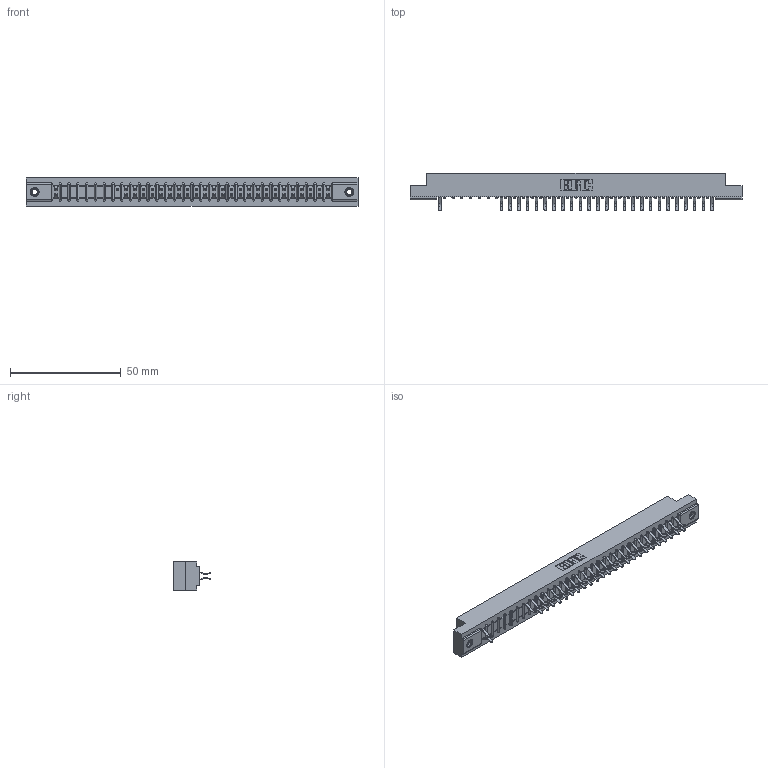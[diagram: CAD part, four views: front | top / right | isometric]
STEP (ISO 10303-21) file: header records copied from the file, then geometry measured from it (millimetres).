
FILE_DESCRIPTION (( 'STEP AP203' ), '1' );
FILE_NAME ('307-064-556-207.STEP', '2018-08-06T10:25:13', ( '' ), ( '' ), 'SwSTEP 2.0', 'SolidWorks 2016', '' );
FILE_SCHEMA (( 'CONFIG_CONTROL_DESIGN' ));
Length unit declared in the file: inch
Products named in the file (4): 307 Part_.156 Dia Mounting Holes; 307-290-001_556; 345-250-001_345-250-005-103; 307-064-556-207
Assembly tree (54 placements, depth 2):
  307-064-556-207
    307 Part_.156 Dia Mounting Holes
    307-290-001_556  x51
    345-250-001_345-250-005-103  x2
Bounding box: 149.81 x 16.97 x 12.7 mm (x, y, z)
Volume: 15668.5 mm3; surface area: 17763.1 mm2
Topology: 54 solids, 54 shells, 2891 faces, 8117 edges, 5246 vertices
Faces by surface type: plane 1863, cylinder 946, sphere 66, cone 12, torus 4
Entity records: 30563 total; most frequent: CARTESIAN_POINT 5042, ORIENTED_EDGE 5002, DIRECTION 4939, EDGE_CURVE 2501, LINE 1913, VECTOR 1913, VERTEX_POINT 1616, AXIS2_PLACEMENT_3D 1513
